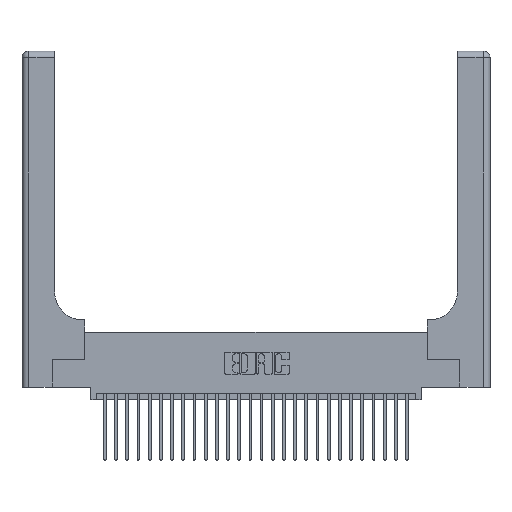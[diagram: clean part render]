
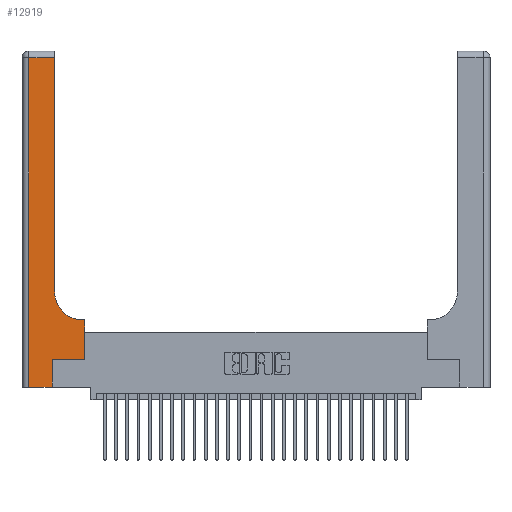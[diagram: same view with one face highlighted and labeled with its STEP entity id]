
A CAD part, top view. The second image highlights one B-rep face of the part: STEP entity #12919.
In plain terms, the highlighted planar face has unit normal (0, 0, 1).
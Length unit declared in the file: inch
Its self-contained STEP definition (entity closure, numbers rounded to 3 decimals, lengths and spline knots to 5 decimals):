
#861 = DIRECTION ( 'NONE',  ( -1., 0., 0. ) ) ;
#1379 = VERTEX_POINT ( 'NONE', #23224 ) ;
#2335 = EDGE_CURVE ( 'NONE', #28755, #3820, #4487, .T. ) ;
#2361 = LINE ( 'NONE', #16999, #24927 ) ;
#2367 = CARTESIAN_POINT ( 'NONE',  ( 0.06, 2.94, 0.37 ) ) ;
#2538 = DIRECTION ( 'NONE',  ( 0., 1., 0. ) ) ;
#2849 = VERTEX_POINT ( 'NONE', #21914 ) ;
#3304 = DIRECTION ( 'NONE',  ( 1., 0., 0. ) ) ;
#3723 = DIRECTION ( 'NONE',  ( -1., 0., 0. ) ) ;
#3820 = VERTEX_POINT ( 'NONE', #21792 ) ;
#3960 = CARTESIAN_POINT ( 'NONE',  ( 0., 0., 0.37 ) ) ;
#4341 = ORIENTED_EDGE ( 'NONE', *, *, #2335, .T. ) ;
#4421 = ORIENTED_EDGE ( 'NONE', *, *, #16811, .T. ) ;
#4487 = LINE ( 'NONE', #11119, #15875 ) ;
#4620 = ORIENTED_EDGE ( 'NONE', *, *, #16604, .T. ) ;
#4773 = EDGE_CURVE ( 'NONE', #12857, #28755, #22911, .T. ) ;
#4809 = LINE ( 'NONE', #19163, #22088 ) ;
#4941 = ORIENTED_EDGE ( 'NONE', *, *, #28172, .T. ) ;
#4947 = ORIENTED_EDGE ( 'NONE', *, *, #11217, .T. ) ;
#4986 = ORIENTED_EDGE ( 'NONE', *, *, #7218, .T. ) ;
#5142 = CARTESIAN_POINT ( 'NONE',  ( 0., 2.94, 0.37 ) ) ;
#5250 = ORIENTED_EDGE ( 'NONE', *, *, #4773, .T. ) ;
#5373 = ORIENTED_EDGE ( 'NONE', *, *, #24175, .T. ) ;
#5432 = ORIENTED_EDGE ( 'NONE', *, *, #6774, .T. ) ;
#5521 = AXIS2_PLACEMENT_3D ( 'NONE', #25650, #14615, #861 ) ;
#5572 = LINE ( 'NONE', #26234, #22786 ) ;
#6063 = CARTESIAN_POINT ( 'NONE',  ( 0.269, 0., 0.37 ) ) ;
#6315 = DIRECTION ( 'NONE',  ( 1., 0., 0. ) ) ;
#6371 = AXIS2_PLACEMENT_3D ( 'NONE', #7813, #23468, #10127 ) ;
#6774 = EDGE_CURVE ( 'NONE', #10880, #12857, #21428, .T. ) ;
#7146 = VECTOR ( 'NONE', #6315, 39.37008 ) ;
#7218 = EDGE_CURVE ( 'NONE', #1379, #29159, #4809, .T. ) ;
#7620 = VERTEX_POINT ( 'NONE', #2367 ) ;
#7813 = CARTESIAN_POINT ( 'NONE',  ( 0.5415, 0.85, 0.37 ) ) ;
#8394 = CARTESIAN_POINT ( 'NONE',  ( 0.2915, 0.6, 0.37 ) ) ;
#10127 = DIRECTION ( 'NONE',  ( 1., 0., 0. ) ) ;
#10240 = VERTEX_POINT ( 'NONE', #6063 ) ;
#10880 = VERTEX_POINT ( 'NONE', #26181 ) ;
#11119 = CARTESIAN_POINT ( 'NONE',  ( 0.2915, 3., 0.37 ) ) ;
#11217 = EDGE_CURVE ( 'NONE', #10240, #1379, #18092, .T. ) ;
#11992 = VECTOR ( 'NONE', #25358, 39.37008 ) ;
#12158 = VECTOR ( 'NONE', #2538, 39.37008 ) ;
#12627 = DIRECTION ( 'NONE',  ( 0., 1., 0. ) ) ;
#12857 = VERTEX_POINT ( 'NONE', #18791 ) ;
#12919 = ADVANCED_FACE ( 'NONE', ( #20545 ), #23429, .F. ) ;
#13968 = CARTESIAN_POINT ( 'NONE',  ( 0.269, 0., 0.37 ) ) ;
#14615 = DIRECTION ( 'NONE',  ( 0., 0., -1. ) ) ;
#15114 = CARTESIAN_POINT ( 'NONE',  ( 0.2915, 0.85, 0.37 ) ) ;
#15202 = DIRECTION ( 'NONE',  ( 0., -1., 0. ) ) ;
#15875 = VECTOR ( 'NONE', #24451, 39.37008 ) ;
#16604 = EDGE_CURVE ( 'NONE', #7620, #2849, #5572, .T. ) ;
#16811 = EDGE_CURVE ( 'NONE', #3820, #7620, #28982, .T. ) ;
#16999 = CARTESIAN_POINT ( 'NONE',  ( 0.5585, 0.25, 0.37 ) ) ;
#18092 = LINE ( 'NONE', #13968, #12158 ) ;
#18791 = CARTESIAN_POINT ( 'NONE',  ( 0.5415, 0.6, 0.37 ) ) ;
#19163 = CARTESIAN_POINT ( 'NONE',  ( 0.269, 0.25, 0.37 ) ) ;
#19728 = CARTESIAN_POINT ( 'NONE',  ( 0.5585, 0.25, 0.37 ) ) ;
#20545 = FACE_OUTER_BOUND ( 'NONE', #21473, .T. ) ;
#21428 = LINE ( 'NONE', #8394, #27979 ) ;
#21473 = EDGE_LOOP ( 'NONE', ( #4341, #4421, #4620, #4941, #4947, #4986, #5373, #5432, #5250 ) ) ;
#21792 = CARTESIAN_POINT ( 'NONE',  ( 0.2915, 2.94, 0.37 ) ) ;
#21914 = CARTESIAN_POINT ( 'NONE',  ( 0.06, 0., 0.37 ) ) ;
#22088 = VECTOR ( 'NONE', #3304, 39.37008 ) ;
#22786 = VECTOR ( 'NONE', #15202, 39.37008 ) ;
#22911 = CIRCLE ( 'NONE', #6371, 0.25 ) ;
#23224 = CARTESIAN_POINT ( 'NONE',  ( 0.269, 0.25, 0.37 ) ) ;
#23429 = PLANE ( 'NONE',  #5521 ) ;
#23468 = DIRECTION ( 'NONE',  ( 0., 0., -1. ) ) ;
#24175 = EDGE_CURVE ( 'NONE', #29159, #10880, #2361, .T. ) ;
#24451 = DIRECTION ( 'NONE',  ( 0., 1., 0. ) ) ;
#24927 = VECTOR ( 'NONE', #12627, 39.37008 ) ;
#25005 = LINE ( 'NONE', #3960, #7146 ) ;
#25358 = DIRECTION ( 'NONE',  ( -1., 0., 0. ) ) ;
#25650 = CARTESIAN_POINT ( 'NONE',  ( 0., 3., 0.37 ) ) ;
#26181 = CARTESIAN_POINT ( 'NONE',  ( 0.5585, 0.6, 0.37 ) ) ;
#26234 = CARTESIAN_POINT ( 'NONE',  ( 0.06, 3., 0.37 ) ) ;
#27979 = VECTOR ( 'NONE', #3723, 39.37008 ) ;
#28172 = EDGE_CURVE ( 'NONE', #2849, #10240, #25005, .T. ) ;
#28755 = VERTEX_POINT ( 'NONE', #15114 ) ;
#28982 = LINE ( 'NONE', #5142, #11992 ) ;
#29159 = VERTEX_POINT ( 'NONE', #19728 ) ;
